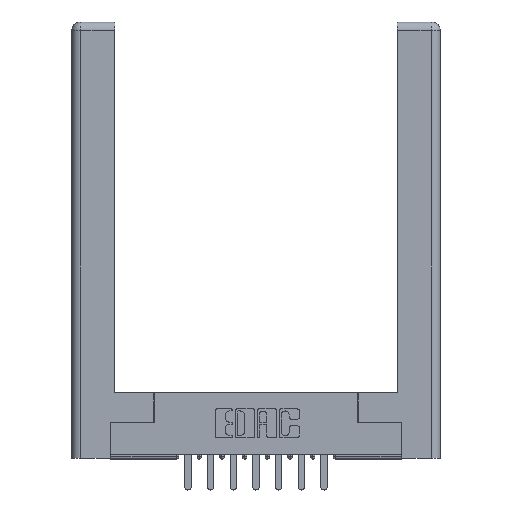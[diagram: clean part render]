
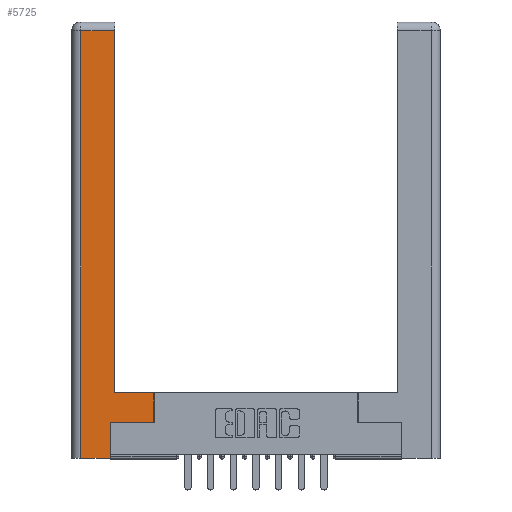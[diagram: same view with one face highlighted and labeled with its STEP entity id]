
A CAD part, top view. The second image highlights one B-rep face of the part: STEP entity #5725.
In plain terms, the highlighted planar face has unit normal (0, 0, 1).
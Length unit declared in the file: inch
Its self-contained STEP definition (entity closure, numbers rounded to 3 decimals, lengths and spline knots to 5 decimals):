
#11 = LINE ( 'NONE', #9454, #9415 ) ;
#321 = ORIENTED_EDGE ( 'NONE', *, *, #3776, .T. ) ;
#503 = CARTESIAN_POINT ( 'NONE',  ( 0.0615, 2.94, 0. ) ) ;
#802 = EDGE_CURVE ( 'NONE', #7585, #2418, #7221, .T. ) ;
#1305 = VECTOR ( 'NONE', #12852, 39.37008 ) ;
#1316 = DIRECTION ( 'NONE',  ( -1., 0., 0. ) ) ;
#2063 = CARTESIAN_POINT ( 'NONE',  ( 0.565, 0.45, 0. ) ) ;
#2283 = VERTEX_POINT ( 'NONE', #4712 ) ;
#2418 = VERTEX_POINT ( 'NONE', #7354 ) ;
#2541 = FACE_OUTER_BOUND ( 'NONE', #9838, .T. ) ;
#2752 = CARTESIAN_POINT ( 'NONE',  ( 0.265, 0., 0. ) ) ;
#2781 = CARTESIAN_POINT ( 'NONE',  ( 0.0615, 2.94, 0. ) ) ;
#3776 = EDGE_CURVE ( 'NONE', #2418, #13360, #8854, .T. ) ;
#3856 = VERTEX_POINT ( 'NONE', #6281 ) ;
#3992 = DIRECTION ( 'NONE',  ( 1., 0., 0. ) ) ;
#4041 = ORIENTED_EDGE ( 'NONE', *, *, #9436, .T. ) ;
#4198 = VERTEX_POINT ( 'NONE', #503 ) ;
#4235 = CARTESIAN_POINT ( 'NONE',  ( 0.265, 0.245, 0. ) ) ;
#4287 = LINE ( 'NONE', #4658, #8855 ) ;
#4395 = CARTESIAN_POINT ( 'NONE',  ( 0.295, 0.45, 0. ) ) ;
#4533 = CARTESIAN_POINT ( 'NONE',  ( 0.295, 2.94, 0. ) ) ;
#4658 = CARTESIAN_POINT ( 'NONE',  ( 0.295, 3., 0. ) ) ;
#4672 = EDGE_CURVE ( 'NONE', #13834, #7585, #12116, .T. ) ;
#4712 = CARTESIAN_POINT ( 'NONE',  ( 0.0615, 0., 0. ) ) ;
#4981 = ORIENTED_EDGE ( 'NONE', *, *, #7576, .T. ) ;
#5121 = LINE ( 'NONE', #2781, #1305 ) ;
#5157 = DIRECTION ( 'NONE',  ( 1., 0., 0. ) ) ;
#5189 = EDGE_CURVE ( 'NONE', #3856, #13834, #12785, .T. ) ;
#5725 = ADVANCED_FACE ( 'NONE', ( #2541 ), #11509, .F. ) ;
#5885 = VECTOR ( 'NONE', #9698, 39.37008 ) ;
#5971 = VECTOR ( 'NONE', #3992, 39.37008 ) ;
#6007 = CARTESIAN_POINT ( 'NONE',  ( 0.565, 0.245, 0. ) ) ;
#6232 = DIRECTION ( 'NONE',  ( 0., -1., 0. ) ) ;
#6281 = CARTESIAN_POINT ( 'NONE',  ( 0.265, 0., 0. ) ) ;
#6924 = ORIENTED_EDGE ( 'NONE', *, *, #11035, .T. ) ;
#7070 = EDGE_CURVE ( 'NONE', #8047, #4198, #5121, .T. ) ;
#7221 = LINE ( 'NONE', #2063, #12733 ) ;
#7289 = CARTESIAN_POINT ( 'NONE',  ( 0.565, 0.245, 0. ) ) ;
#7354 = CARTESIAN_POINT ( 'NONE',  ( 0.565, 0.45, 0. ) ) ;
#7528 = DIRECTION ( 'NONE',  ( 0., 1., 0. ) ) ;
#7576 = EDGE_CURVE ( 'NONE', #2283, #3856, #10491, .T. ) ;
#7585 = VERTEX_POINT ( 'NONE', #7289 ) ;
#7707 = ORIENTED_EDGE ( 'NONE', *, *, #7070, .T. ) ;
#8047 = VERTEX_POINT ( 'NONE', #4533 ) ;
#8691 = ORIENTED_EDGE ( 'NONE', *, *, #802, .T. ) ;
#8854 = LINE ( 'NONE', #13093, #5885 ) ;
#8855 = VECTOR ( 'NONE', #12420, 39.37008 ) ;
#8996 = VECTOR ( 'NONE', #13161, 39.37008 ) ;
#9200 = VECTOR ( 'NONE', #5157, 39.37008 ) ;
#9415 = VECTOR ( 'NONE', #6232, 39.37008 ) ;
#9436 = EDGE_CURVE ( 'NONE', #4198, #2283, #11, .T. ) ;
#9454 = CARTESIAN_POINT ( 'NONE',  ( 0.0615, 0., 0. ) ) ;
#9678 = CARTESIAN_POINT ( 'NONE',  ( 0.265, 0.245, 0. ) ) ;
#9698 = DIRECTION ( 'NONE',  ( -1., 0., 0. ) ) ;
#9838 = EDGE_LOOP ( 'NONE', ( #6924, #7707, #4041, #4981, #9919, #10662, #8691, #321 ) ) ;
#9919 = ORIENTED_EDGE ( 'NONE', *, *, #5189, .T. ) ;
#10491 = LINE ( 'NONE', #2752, #5971 ) ;
#10662 = ORIENTED_EDGE ( 'NONE', *, *, #4672, .T. ) ;
#11035 = EDGE_CURVE ( 'NONE', #13360, #8047, #4287, .T. ) ;
#11374 = DIRECTION ( 'NONE',  ( 0., 0., -1. ) ) ;
#11509 = PLANE ( 'NONE',  #12204 ) ;
#12116 = LINE ( 'NONE', #6007, #9200 ) ;
#12204 = AXIS2_PLACEMENT_3D ( 'NONE', #12373, #11374, #1316 ) ;
#12373 = CARTESIAN_POINT ( 'NONE',  ( 0., 0., 0. ) ) ;
#12420 = DIRECTION ( 'NONE',  ( 0., 1., 0. ) ) ;
#12733 = VECTOR ( 'NONE', #7528, 39.37008 ) ;
#12785 = LINE ( 'NONE', #4235, #8996 ) ;
#12852 = DIRECTION ( 'NONE',  ( -1., 0., 0. ) ) ;
#13093 = CARTESIAN_POINT ( 'NONE',  ( 0.295, 0.45, 0. ) ) ;
#13161 = DIRECTION ( 'NONE',  ( 0., 1., 0. ) ) ;
#13360 = VERTEX_POINT ( 'NONE', #4395 ) ;
#13834 = VERTEX_POINT ( 'NONE', #9678 ) ;
